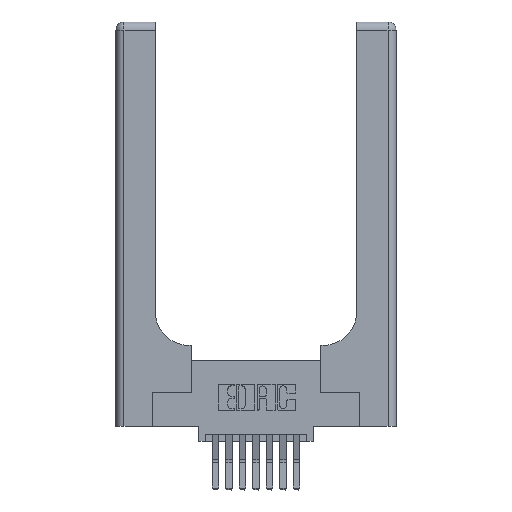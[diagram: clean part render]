
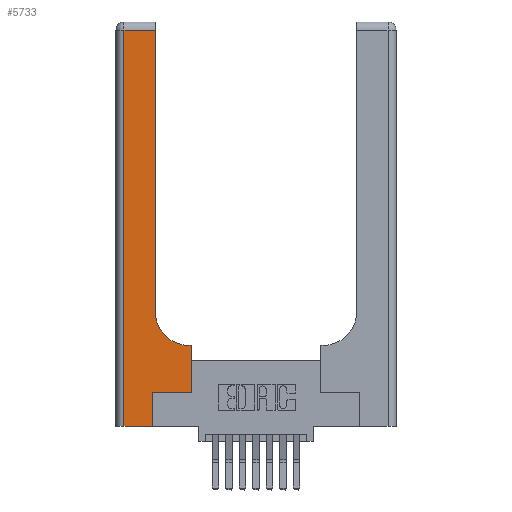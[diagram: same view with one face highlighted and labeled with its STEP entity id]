
A CAD part, top view. The second image highlights one B-rep face of the part: STEP entity #5733.
In plain terms, the highlighted planar face has unit normal (0, 0, 1).
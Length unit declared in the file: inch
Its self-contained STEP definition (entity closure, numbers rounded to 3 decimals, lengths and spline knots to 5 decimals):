
#138 = ORIENTED_EDGE ( 'NONE', *, *, #14417, .T. ) ;
#217 = CARTESIAN_POINT ( 'NONE',  ( 0.269, 0.25, 0.37 ) ) ;
#320 = ORIENTED_EDGE ( 'NONE', *, *, #3781, .T. ) ;
#617 = LINE ( 'NONE', #2190, #10764 ) ;
#712 = AXIS2_PLACEMENT_3D ( 'NONE', #5552, #14075, #3188 ) ;
#898 = DIRECTION ( 'NONE',  ( 0., 0., -1. ) ) ;
#1422 = CARTESIAN_POINT ( 'NONE',  ( 0.5415, 0.6, 0.37 ) ) ;
#1867 = CARTESIAN_POINT ( 'NONE',  ( 0.06, 2.94, 0.37 ) ) ;
#1995 = ORIENTED_EDGE ( 'NONE', *, *, #5724, .T. ) ;
#2021 = CARTESIAN_POINT ( 'NONE',  ( 0., 3., 0.37 ) ) ;
#2129 = CIRCLE ( 'NONE', #712, 0.25 ) ;
#2190 = CARTESIAN_POINT ( 'NONE',  ( 0.06, 3., 0.37 ) ) ;
#2207 = DIRECTION ( 'NONE',  ( 0., 1., 0. ) ) ;
#2674 = CARTESIAN_POINT ( 'NONE',  ( 0.5585, 0.25, 0.37 ) ) ;
#2839 = DIRECTION ( 'NONE',  ( 0., 1., 0. ) ) ;
#2950 = FACE_OUTER_BOUND ( 'NONE', #6210, .T. ) ;
#3188 = DIRECTION ( 'NONE',  ( 1., 0., 0. ) ) ;
#3781 = EDGE_CURVE ( 'NONE', #13199, #15043, #617, .T. ) ;
#4434 = EDGE_CURVE ( 'NONE', #12381, #13199, #9019, .T. ) ;
#4609 = ORIENTED_EDGE ( 'NONE', *, *, #9918, .T. ) ;
#5232 = VECTOR ( 'NONE', #8459, 39.37008 ) ;
#5552 = CARTESIAN_POINT ( 'NONE',  ( 0.5415, 0.85, 0.37 ) ) ;
#5724 = EDGE_CURVE ( 'NONE', #15043, #12648, #9379, .T. ) ;
#5733 = ADVANCED_FACE ( 'NONE', ( #2950 ), #6690, .F. ) ;
#5739 = ORIENTED_EDGE ( 'NONE', *, *, #4434, .T. ) ;
#5857 = VECTOR ( 'NONE', #2207, 39.37008 ) ;
#6210 = EDGE_LOOP ( 'NONE', ( #10484, #5739, #320, #1995, #9654, #4609, #11045, #138, #8277 ) ) ;
#6264 = CARTESIAN_POINT ( 'NONE',  ( 0.2915, 0.85, 0.37 ) ) ;
#6371 = VERTEX_POINT ( 'NONE', #1422 ) ;
#6543 = DIRECTION ( 'NONE',  ( 0., 1., 0. ) ) ;
#6601 = CARTESIAN_POINT ( 'NONE',  ( 0.2915, 0.6, 0.37 ) ) ;
#6616 = VERTEX_POINT ( 'NONE', #7997 ) ;
#6625 = CARTESIAN_POINT ( 'NONE',  ( 0.5585, 0.25, 0.37 ) ) ;
#6690 = PLANE ( 'NONE',  #12531 ) ;
#7192 = VECTOR ( 'NONE', #7791, 39.37008 ) ;
#7328 = EDGE_CURVE ( 'NONE', #7513, #6616, #15161, .T. ) ;
#7513 = VERTEX_POINT ( 'NONE', #6625 ) ;
#7609 = CARTESIAN_POINT ( 'NONE',  ( 0.269, 0., 0.37 ) ) ;
#7791 = DIRECTION ( 'NONE',  ( -1., 0., 0. ) ) ;
#7886 = DIRECTION ( 'NONE',  ( -1., 0., 0. ) ) ;
#7997 = CARTESIAN_POINT ( 'NONE',  ( 0.5585, 0.6, 0.37 ) ) ;
#8277 = ORIENTED_EDGE ( 'NONE', *, *, #15285, .T. ) ;
#8459 = DIRECTION ( 'NONE',  ( 1., 0., 0. ) ) ;
#8510 = CARTESIAN_POINT ( 'NONE',  ( 0.2915, 2.94, 0.37 ) ) ;
#8586 = EDGE_CURVE ( 'NONE', #12525, #12381, #9088, .T. ) ;
#8715 = VECTOR ( 'NONE', #6543, 39.37008 ) ;
#9019 = LINE ( 'NONE', #11291, #10547 ) ;
#9088 = LINE ( 'NONE', #13011, #5857 ) ;
#9124 = CARTESIAN_POINT ( 'NONE',  ( 0.06, 0., 0.37 ) ) ;
#9379 = LINE ( 'NONE', #11530, #13341 ) ;
#9654 = ORIENTED_EDGE ( 'NONE', *, *, #12234, .T. ) ;
#9918 = EDGE_CURVE ( 'NONE', #11586, #7513, #14930, .T. ) ;
#10024 = VECTOR ( 'NONE', #2839, 39.37008 ) ;
#10484 = ORIENTED_EDGE ( 'NONE', *, *, #8586, .T. ) ;
#10547 = VECTOR ( 'NONE', #11235, 39.37008 ) ;
#10764 = VECTOR ( 'NONE', #11683, 39.37008 ) ;
#11045 = ORIENTED_EDGE ( 'NONE', *, *, #7328, .T. ) ;
#11235 = DIRECTION ( 'NONE',  ( -1., 0., 0. ) ) ;
#11291 = CARTESIAN_POINT ( 'NONE',  ( 0., 2.94, 0.37 ) ) ;
#11530 = CARTESIAN_POINT ( 'NONE',  ( 0., 0., 0.37 ) ) ;
#11586 = VERTEX_POINT ( 'NONE', #13940 ) ;
#11683 = DIRECTION ( 'NONE',  ( 0., -1., 0. ) ) ;
#12234 = EDGE_CURVE ( 'NONE', #12648, #11586, #13471, .T. ) ;
#12381 = VERTEX_POINT ( 'NONE', #8510 ) ;
#12525 = VERTEX_POINT ( 'NONE', #6264 ) ;
#12531 = AXIS2_PLACEMENT_3D ( 'NONE', #2021, #898, #7886 ) ;
#12648 = VERTEX_POINT ( 'NONE', #7609 ) ;
#12737 = DIRECTION ( 'NONE',  ( 1., 0., 0. ) ) ;
#13011 = CARTESIAN_POINT ( 'NONE',  ( 0.2915, 3., 0.37 ) ) ;
#13199 = VERTEX_POINT ( 'NONE', #1867 ) ;
#13341 = VECTOR ( 'NONE', #12737, 39.37008 ) ;
#13471 = LINE ( 'NONE', #13821, #8715 ) ;
#13663 = LINE ( 'NONE', #6601, #7192 ) ;
#13821 = CARTESIAN_POINT ( 'NONE',  ( 0.269, 0., 0.37 ) ) ;
#13940 = CARTESIAN_POINT ( 'NONE',  ( 0.269, 0.25, 0.37 ) ) ;
#14075 = DIRECTION ( 'NONE',  ( 0., 0., -1. ) ) ;
#14417 = EDGE_CURVE ( 'NONE', #6616, #6371, #13663, .T. ) ;
#14930 = LINE ( 'NONE', #217, #5232 ) ;
#15043 = VERTEX_POINT ( 'NONE', #9124 ) ;
#15161 = LINE ( 'NONE', #2674, #10024 ) ;
#15285 = EDGE_CURVE ( 'NONE', #6371, #12525, #2129, .T. ) ;
